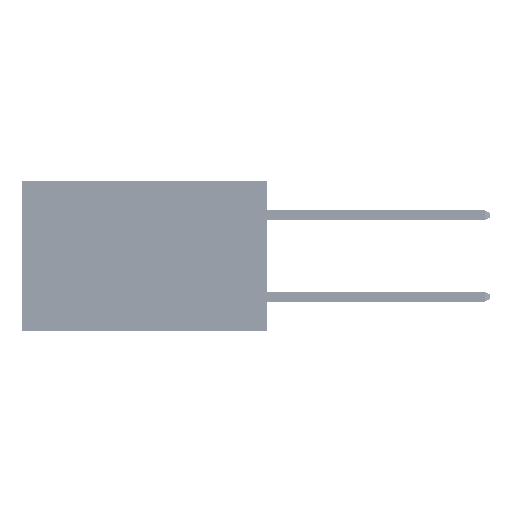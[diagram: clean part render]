
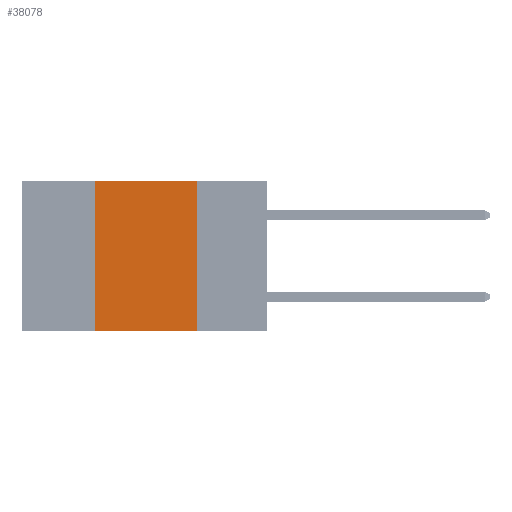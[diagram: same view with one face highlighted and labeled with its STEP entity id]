
A CAD part, left-side view. The second image highlights one B-rep face of the part: STEP entity #38078.
In plain terms, the highlighted planar face has unit normal (-1, 0, 0).
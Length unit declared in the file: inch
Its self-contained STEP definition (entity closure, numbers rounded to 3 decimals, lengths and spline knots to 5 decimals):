
#1030 = ORIENTED_EDGE ( 'NONE', *, *, #31152, .F. ) ;
#2369 = VERTEX_POINT ( 'NONE', #46096 ) ;
#3797 = CARTESIAN_POINT ( 'NONE',  ( 0., 0.17, 0. ) ) ;
#6218 = EDGE_CURVE ( 'NONE', #6812, #37559, #7520, .T. ) ;
#6812 = VERTEX_POINT ( 'NONE', #14822 ) ;
#7520 = LINE ( 'NONE', #35799, #31584 ) ;
#9182 = EDGE_CURVE ( 'NONE', #6812, #2369, #43719, .T. ) ;
#11721 = AXIS2_PLACEMENT_3D ( 'NONE', #25990, #34720, #22361 ) ;
#14822 = CARTESIAN_POINT ( 'NONE',  ( 0., 0.42, -0.37 ) ) ;
#16110 = DIRECTION ( 'NONE',  ( 0., 0., -1. ) ) ;
#18463 = ORIENTED_EDGE ( 'NONE', *, *, #9182, .F. ) ;
#22106 = EDGE_CURVE ( 'NONE', #45917, #37559, #29099, .T. ) ;
#22361 = DIRECTION ( 'NONE',  ( 0., 0., -1. ) ) ;
#23287 = VECTOR ( 'NONE', #16110, 39.37008 ) ;
#23710 = CARTESIAN_POINT ( 'NONE',  ( 0., 0.17, -0.37 ) ) ;
#25619 = CARTESIAN_POINT ( 'NONE',  ( 0., 0.42, 0. ) ) ;
#25990 = CARTESIAN_POINT ( 'NONE',  ( 0., 0.6, 0. ) ) ;
#27029 = LINE ( 'NONE', #37936, #36786 ) ;
#29099 = LINE ( 'NONE', #3797, #23287 ) ;
#30394 = CARTESIAN_POINT ( 'NONE',  ( 0., 0.17, 0. ) ) ;
#31152 = EDGE_CURVE ( 'NONE', #2369, #45917, #27029, .T. ) ;
#31584 = VECTOR ( 'NONE', #32307, 39.37008 ) ;
#31666 = EDGE_LOOP ( 'NONE', ( #51074, #1030, #18463, #51027 ) ) ;
#32307 = DIRECTION ( 'NONE',  ( 0., -1., 0. ) ) ;
#33558 = DIRECTION ( 'NONE',  ( 0., -1., 0. ) ) ;
#34720 = DIRECTION ( 'NONE',  ( 1., 0., 0. ) ) ;
#34762 = FACE_OUTER_BOUND ( 'NONE', #31666, .T. ) ;
#35799 = CARTESIAN_POINT ( 'NONE',  ( 0., 0.6, -0.37 ) ) ;
#36786 = VECTOR ( 'NONE', #33558, 39.37008 ) ;
#37559 = VERTEX_POINT ( 'NONE', #23710 ) ;
#37936 = CARTESIAN_POINT ( 'NONE',  ( 0., 0.6, 0. ) ) ;
#38078 = ADVANCED_FACE ( 'NONE', ( #34762 ), #43098, .F. ) ;
#42912 = DIRECTION ( 'NONE',  ( 0., 0., 1. ) ) ;
#43098 = PLANE ( 'NONE',  #11721 ) ;
#43719 = LINE ( 'NONE', #25619, #50864 ) ;
#45917 = VERTEX_POINT ( 'NONE', #30394 ) ;
#46096 = CARTESIAN_POINT ( 'NONE',  ( 0., 0.42, 0. ) ) ;
#50864 = VECTOR ( 'NONE', #42912, 39.37008 ) ;
#51027 = ORIENTED_EDGE ( 'NONE', *, *, #6218, .T. ) ;
#51074 = ORIENTED_EDGE ( 'NONE', *, *, #22106, .F. ) ;
